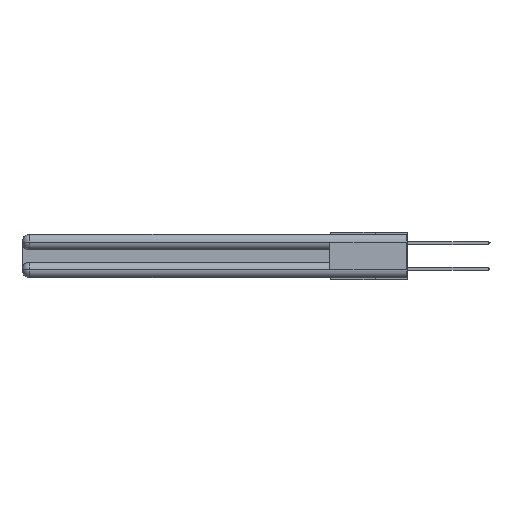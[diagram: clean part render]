
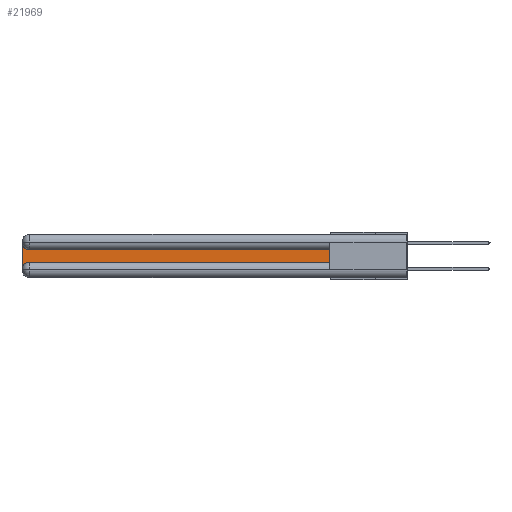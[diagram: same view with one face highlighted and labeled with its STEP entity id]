
A CAD part, left-side view. The second image highlights one B-rep face of the part: STEP entity #21969.
In plain terms, the highlighted planar face has unit normal (-1, 0, 0).
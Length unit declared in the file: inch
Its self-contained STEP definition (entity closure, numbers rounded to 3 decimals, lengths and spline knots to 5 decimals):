
#34 = CARTESIAN_POINT ( 'NONE',  ( 0.075, 2.94, -0.0625 ) ) ;
#491 = VECTOR ( 'NONE', #31075, 39.37008 ) ;
#2054 = ORIENTED_EDGE ( 'NONE', *, *, #12812, .T. ) ;
#2297 = CARTESIAN_POINT ( 'NONE',  ( 0.075, 2.94, -0.2175 ) ) ;
#2449 = CARTESIAN_POINT ( 'NONE',  ( 0.075, 0.6, -0.2175 ) ) ;
#3464 = AXIS2_PLACEMENT_3D ( 'NONE', #34, #14968, #17458 ) ;
#3642 = CARTESIAN_POINT ( 'NONE',  ( 0.075, 3., -0.2175 ) ) ;
#4026 = LINE ( 'NONE', #3642, #16407 ) ;
#4180 = FACE_OUTER_BOUND ( 'NONE', #4683, .T. ) ;
#4234 = VERTEX_POINT ( 'NONE', #2297 ) ;
#4683 = EDGE_LOOP ( 'NONE', ( #25587, #28642, #8574, #2054, #6526, #6630 ) ) ;
#5984 = DIRECTION ( 'NONE',  ( 1., 0., 0. ) ) ;
#6120 = VECTOR ( 'NONE', #19524, 39.37008 ) ;
#6231 = CARTESIAN_POINT ( 'NONE',  ( 0.075, 0.6, -0.2175 ) ) ;
#6526 = ORIENTED_EDGE ( 'NONE', *, *, #14141, .T. ) ;
#6630 = ORIENTED_EDGE ( 'NONE', *, *, #22730, .T. ) ;
#7560 = VERTEX_POINT ( 'NONE', #2449 ) ;
#7983 = LINE ( 'NONE', #9748, #6120 ) ;
#8574 = ORIENTED_EDGE ( 'NONE', *, *, #18675, .T. ) ;
#9369 = CARTESIAN_POINT ( 'NONE',  ( 0.075, 3., -0.2775 ) ) ;
#9748 = CARTESIAN_POINT ( 'NONE',  ( 0.075, 0.6, -0.1225 ) ) ;
#9930 = VERTEX_POINT ( 'NONE', #9369 ) ;
#10508 = CARTESIAN_POINT ( 'NONE',  ( 0.075, 2.94, -0.2775 ) ) ;
#11319 = DIRECTION ( 'NONE',  ( 0., 0., -1. ) ) ;
#11353 = CARTESIAN_POINT ( 'NONE',  ( 0.075, 2.94, -0.1225 ) ) ;
#11762 = CARTESIAN_POINT ( 'NONE',  ( 0.075, 0.6, -0.1225 ) ) ;
#12006 = CARTESIAN_POINT ( 'NONE',  ( 0.075, 3., -0.1225 ) ) ;
#12812 = EDGE_CURVE ( 'NONE', #9930, #4234, #14906, .T. ) ;
#13024 = DIRECTION ( 'NONE',  ( 0., 0., -1. ) ) ;
#14141 = EDGE_CURVE ( 'NONE', #4234, #7560, #23319, .T. ) ;
#14703 = CARTESIAN_POINT ( 'NONE',  ( 0.075, 0.6, -0.2175 ) ) ;
#14906 = CIRCLE ( 'NONE', #26187, 0.06 ) ;
#14968 = DIRECTION ( 'NONE',  ( 1., 0., 0. ) ) ;
#15164 = CARTESIAN_POINT ( 'NONE',  ( 0.075, 3., -0.0625 ) ) ;
#16407 = VECTOR ( 'NONE', #11319, 39.37008 ) ;
#16590 = LINE ( 'NONE', #14703, #25140 ) ;
#16847 = PLANE ( 'NONE',  #28563 ) ;
#17458 = DIRECTION ( 'NONE',  ( 0., 0., -1. ) ) ;
#18106 = VERTEX_POINT ( 'NONE', #15164 ) ;
#18675 = EDGE_CURVE ( 'NONE', #18106, #9930, #4026, .T. ) ;
#19524 = DIRECTION ( 'NONE',  ( 0., 1., 0. ) ) ;
#20846 = VERTEX_POINT ( 'NONE', #11353 ) ;
#21969 = ADVANCED_FACE ( 'NONE', ( #4180 ), #16847, .F. ) ;
#22730 = EDGE_CURVE ( 'NONE', #7560, #31247, #16590, .T. ) ;
#23319 = LINE ( 'NONE', #6231, #491 ) ;
#23889 = EDGE_CURVE ( 'NONE', #31247, #20846, #7983, .T. ) ;
#23891 = CIRCLE ( 'NONE', #3464, 0.06 ) ;
#24443 = DIRECTION ( 'NONE',  ( 0., 0., -1. ) ) ;
#25140 = VECTOR ( 'NONE', #27023, 39.37008 ) ;
#25587 = ORIENTED_EDGE ( 'NONE', *, *, #23889, .T. ) ;
#26187 = AXIS2_PLACEMENT_3D ( 'NONE', #10508, #5984, #13024 ) ;
#27023 = DIRECTION ( 'NONE',  ( 0., 0., 1. ) ) ;
#28563 = AXIS2_PLACEMENT_3D ( 'NONE', #12006, #29277, #24443 ) ;
#28642 = ORIENTED_EDGE ( 'NONE', *, *, #30528, .T. ) ;
#29277 = DIRECTION ( 'NONE',  ( 1., 0., 0. ) ) ;
#30528 = EDGE_CURVE ( 'NONE', #20846, #18106, #23891, .T. ) ;
#31075 = DIRECTION ( 'NONE',  ( 0., -1., 0. ) ) ;
#31247 = VERTEX_POINT ( 'NONE', #11762 ) ;
